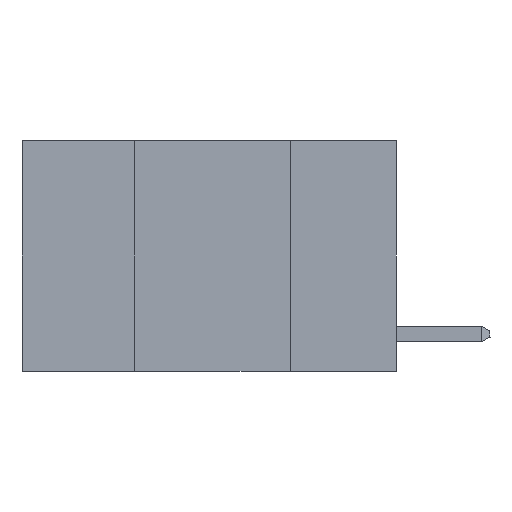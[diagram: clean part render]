
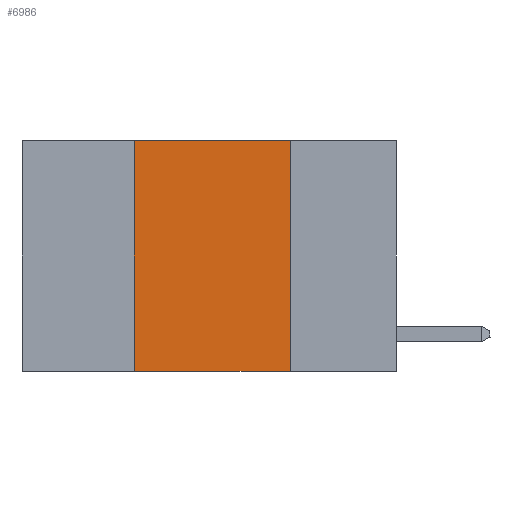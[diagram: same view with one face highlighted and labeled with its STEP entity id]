
A CAD part, left-side view. The second image highlights one B-rep face of the part: STEP entity #6986.
In plain terms, the highlighted planar face has unit normal (-1, 0, 0).
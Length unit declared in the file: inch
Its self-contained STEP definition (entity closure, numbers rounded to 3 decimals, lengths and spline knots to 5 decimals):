
#265 = VERTEX_POINT ( 'NONE', #6334 ) ;
#710 = VECTOR ( 'NONE', #12358, 39.37008 ) ;
#1244 = PLANE ( 'NONE',  #8570 ) ;
#1334 = LINE ( 'NONE', #2659, #9929 ) ;
#1349 = CARTESIAN_POINT ( 'NONE',  ( 0., 0.6, -0.37 ) ) ;
#1363 = EDGE_CURVE ( 'NONE', #12324, #265, #1334, .T. ) ;
#1399 = CARTESIAN_POINT ( 'NONE',  ( 0., 0.42, 0. ) ) ;
#1465 = LINE ( 'NONE', #12848, #11226 ) ;
#1693 = DIRECTION ( 'NONE',  ( 0., 0., 1. ) ) ;
#1916 = CARTESIAN_POINT ( 'NONE',  ( 0., 0.42, 0. ) ) ;
#1944 = CARTESIAN_POINT ( 'NONE',  ( 0., 0.17, -0.37 ) ) ;
#2540 = CARTESIAN_POINT ( 'NONE',  ( 0., 0.42, -0.37 ) ) ;
#2608 = VERTEX_POINT ( 'NONE', #2540 ) ;
#2659 = CARTESIAN_POINT ( 'NONE',  ( 0., 0.6, 0. ) ) ;
#3226 = EDGE_LOOP ( 'NONE', ( #14504, #4738, #12299, #9057 ) ) ;
#4738 = ORIENTED_EDGE ( 'NONE', *, *, #1363, .F. ) ;
#6334 = CARTESIAN_POINT ( 'NONE',  ( 0., 0.17, 0. ) ) ;
#6890 = DIRECTION ( 'NONE',  ( 0., 0., -1. ) ) ;
#6903 = DIRECTION ( 'NONE',  ( 0., -1., 0. ) ) ;
#6986 = ADVANCED_FACE ( 'NONE', ( #10258 ), #1244, .F. ) ;
#7030 = CARTESIAN_POINT ( 'NONE',  ( 0., 0.6, 0. ) ) ;
#7987 = EDGE_CURVE ( 'NONE', #2608, #12324, #13143, .T. ) ;
#8321 = VECTOR ( 'NONE', #1693, 39.37008 ) ;
#8570 = AXIS2_PLACEMENT_3D ( 'NONE', #7030, #9297, #12545 ) ;
#8652 = VERTEX_POINT ( 'NONE', #1944 ) ;
#9057 = ORIENTED_EDGE ( 'NONE', *, *, #14266, .T. ) ;
#9297 = DIRECTION ( 'NONE',  ( 1., 0., 0. ) ) ;
#9929 = VECTOR ( 'NONE', #6903, 39.37008 ) ;
#10258 = FACE_OUTER_BOUND ( 'NONE', #3226, .T. ) ;
#11226 = VECTOR ( 'NONE', #6890, 39.37008 ) ;
#12214 = LINE ( 'NONE', #1349, #710 ) ;
#12299 = ORIENTED_EDGE ( 'NONE', *, *, #7987, .F. ) ;
#12310 = EDGE_CURVE ( 'NONE', #265, #8652, #1465, .T. ) ;
#12324 = VERTEX_POINT ( 'NONE', #1399 ) ;
#12358 = DIRECTION ( 'NONE',  ( 0., -1., 0. ) ) ;
#12545 = DIRECTION ( 'NONE',  ( 0., 0., -1. ) ) ;
#12848 = CARTESIAN_POINT ( 'NONE',  ( 0., 0.17, 0. ) ) ;
#13143 = LINE ( 'NONE', #1916, #8321 ) ;
#14266 = EDGE_CURVE ( 'NONE', #2608, #8652, #12214, .T. ) ;
#14504 = ORIENTED_EDGE ( 'NONE', *, *, #12310, .F. ) ;
